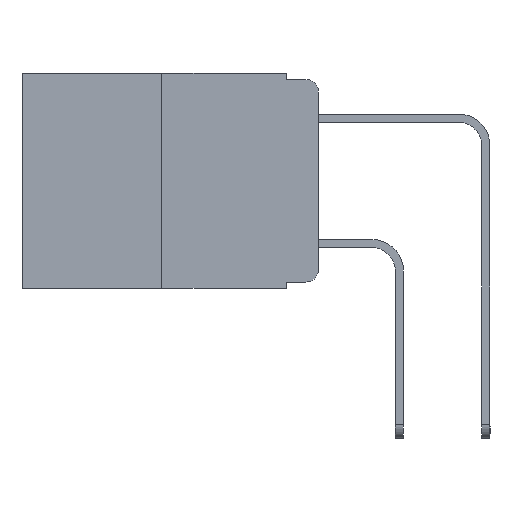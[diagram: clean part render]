
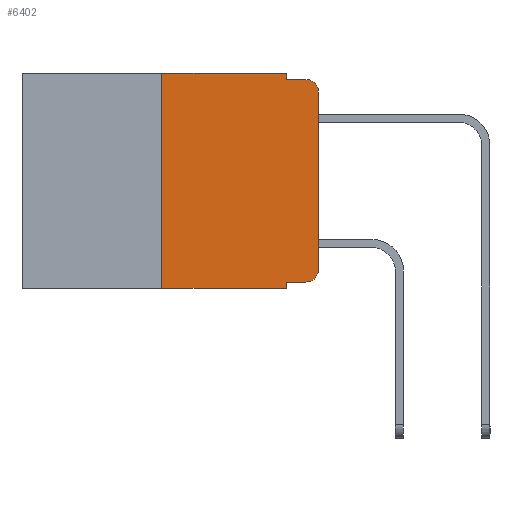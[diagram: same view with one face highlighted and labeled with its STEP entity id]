
A CAD part, left-side view. The second image highlights one B-rep face of the part: STEP entity #6402.
In plain terms, the highlighted planar face has unit normal (-1, 0, 0).
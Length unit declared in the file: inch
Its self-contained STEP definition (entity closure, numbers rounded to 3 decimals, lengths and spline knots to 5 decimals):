
#211 = VERTEX_POINT ( 'NONE', #11814 ) ;
#403 = ORIENTED_EDGE ( 'NONE', *, *, #9901, .F. ) ;
#454 = CARTESIAN_POINT ( 'NONE',  ( 0., 0.051, -0.333 ) ) ;
#734 = DIRECTION ( 'NONE',  ( -1., 0., 0. ) ) ;
#766 = EDGE_CURVE ( 'NONE', #15834, #3114, #13687, .T. ) ;
#1026 = VECTOR ( 'NONE', #3762, 39.37008 ) ;
#1349 = VECTOR ( 'NONE', #5720, 39.37008 ) ;
#1378 = CARTESIAN_POINT ( 'NONE',  ( 0., 0., -0.03 ) ) ;
#1543 = DIRECTION ( 'NONE',  ( -1., 0., 0. ) ) ;
#2592 = VERTEX_POINT ( 'NONE', #6957 ) ;
#2936 = ORIENTED_EDGE ( 'NONE', *, *, #7957, .F. ) ;
#3085 = DIRECTION ( 'NONE',  ( 1., 0., 0. ) ) ;
#3114 = VERTEX_POINT ( 'NONE', #5483 ) ;
#3618 = VERTEX_POINT ( 'NONE', #7188 ) ;
#3762 = DIRECTION ( 'NONE',  ( 0., 0., 1. ) ) ;
#3896 = VECTOR ( 'NONE', #9650, 39.37008 ) ;
#3955 = EDGE_CURVE ( 'NONE', #3114, #6745, #17941, .T. ) ;
#4004 = EDGE_CURVE ( 'NONE', #13956, #15834, #19789, .T. ) ;
#4107 = DIRECTION ( 'NONE',  ( 0., 0., 1. ) ) ;
#4834 = CARTESIAN_POINT ( 'NONE',  ( 0., 0.02, -0.03 ) ) ;
#5006 = VERTEX_POINT ( 'NONE', #10937 ) ;
#5483 = CARTESIAN_POINT ( 'NONE',  ( 0., 0., -0.313 ) ) ;
#5720 = DIRECTION ( 'NONE',  ( 0., -1., 0. ) ) ;
#5876 = ORIENTED_EDGE ( 'NONE', *, *, #15227, .F. ) ;
#6144 = EDGE_CURVE ( 'NONE', #3618, #10780, #10019, .T. ) ;
#6225 = ORIENTED_EDGE ( 'NONE', *, *, #6144, .T. ) ;
#6402 = ADVANCED_FACE ( 'NONE', ( #9275 ), #20260, .F. ) ;
#6668 = AXIS2_PLACEMENT_3D ( 'NONE', #4834, #1543, #14152 ) ;
#6745 = VERTEX_POINT ( 'NONE', #1378 ) ;
#6957 = CARTESIAN_POINT ( 'NONE',  ( 0., 0.25, 0. ) ) ;
#7032 = ORIENTED_EDGE ( 'NONE', *, *, #3955, .T. ) ;
#7151 = CARTESIAN_POINT ( 'NONE',  ( 0., 0.051, -0.343 ) ) ;
#7162 = CARTESIAN_POINT ( 'NONE',  ( 0., 0.051, -0.333 ) ) ;
#7188 = CARTESIAN_POINT ( 'NONE',  ( 0., 0.25, -0.343 ) ) ;
#7580 = CARTESIAN_POINT ( 'NONE',  ( 0., 0.051, 0. ) ) ;
#7642 = CIRCLE ( 'NONE', #6668, 0.02 ) ;
#7763 = ORIENTED_EDGE ( 'NONE', *, *, #17057, .F. ) ;
#7957 = EDGE_CURVE ( 'NONE', #211, #5006, #18241, .T. ) ;
#8257 = VECTOR ( 'NONE', #8454, 39.37008 ) ;
#8454 = DIRECTION ( 'NONE',  ( 0., -1., 0. ) ) ;
#8657 = CARTESIAN_POINT ( 'NONE',  ( 0., 0.473, 0. ) ) ;
#9275 = FACE_OUTER_BOUND ( 'NONE', #9461, .T. ) ;
#9461 = EDGE_LOOP ( 'NONE', ( #7032, #16807, #2936, #19501, #403, #5876, #6225, #7763, #18917, #9912 ) ) ;
#9650 = DIRECTION ( 'NONE',  ( 0., 0., -1. ) ) ;
#9901 = EDGE_CURVE ( 'NONE', #2592, #14738, #19431, .T. ) ;
#9912 = ORIENTED_EDGE ( 'NONE', *, *, #766, .T. ) ;
#10019 = LINE ( 'NONE', #19439, #10185 ) ;
#10185 = VECTOR ( 'NONE', #14489, 39.37008 ) ;
#10679 = CARTESIAN_POINT ( 'NONE',  ( 0., 0.051, -0.01 ) ) ;
#10780 = VERTEX_POINT ( 'NONE', #7151 ) ;
#10937 = CARTESIAN_POINT ( 'NONE',  ( 0., 0.02, -0.01 ) ) ;
#11277 = CARTESIAN_POINT ( 'NONE',  ( 0., 0.02, -0.333 ) ) ;
#11814 = CARTESIAN_POINT ( 'NONE',  ( 0., 0.051, -0.01 ) ) ;
#12281 = CARTESIAN_POINT ( 'NONE',  ( 0., 0.25, 0. ) ) ;
#12687 = AXIS2_PLACEMENT_3D ( 'NONE', #13659, #734, #19656 ) ;
#12873 = EDGE_CURVE ( 'NONE', #6745, #5006, #7642, .T. ) ;
#13001 = VECTOR ( 'NONE', #13585, 39.37008 ) ;
#13506 = DIRECTION ( 'NONE',  ( 0., 0., -1. ) ) ;
#13585 = DIRECTION ( 'NONE',  ( 0., -1., 0. ) ) ;
#13659 = CARTESIAN_POINT ( 'NONE',  ( 0., 0.02, -0.313 ) ) ;
#13687 = CIRCLE ( 'NONE', #12687, 0.02 ) ;
#13956 = VERTEX_POINT ( 'NONE', #454 ) ;
#14152 = DIRECTION ( 'NONE',  ( 0., 0., -1. ) ) ;
#14433 = CARTESIAN_POINT ( 'NONE',  ( 0., 0.051, 0. ) ) ;
#14489 = DIRECTION ( 'NONE',  ( 0., -1., 0. ) ) ;
#14738 = VERTEX_POINT ( 'NONE', #16021 ) ;
#15227 = EDGE_CURVE ( 'NONE', #3618, #2592, #16741, .T. ) ;
#15397 = DIRECTION ( 'NONE',  ( 0., 0., -1. ) ) ;
#15834 = VERTEX_POINT ( 'NONE', #11277 ) ;
#16021 = CARTESIAN_POINT ( 'NONE',  ( 0., 0.051, 0. ) ) ;
#16741 = LINE ( 'NONE', #12281, #18035 ) ;
#16807 = ORIENTED_EDGE ( 'NONE', *, *, #12873, .T. ) ;
#17057 = EDGE_CURVE ( 'NONE', #13956, #10780, #18372, .T. ) ;
#17173 = EDGE_CURVE ( 'NONE', #14738, #211, #18667, .T. ) ;
#17941 = LINE ( 'NONE', #19281, #1026 ) ;
#18035 = VECTOR ( 'NONE', #4107, 39.37008 ) ;
#18241 = LINE ( 'NONE', #10679, #13001 ) ;
#18372 = LINE ( 'NONE', #7580, #19097 ) ;
#18667 = LINE ( 'NONE', #14433, #3896 ) ;
#18917 = ORIENTED_EDGE ( 'NONE', *, *, #4004, .T. ) ;
#19097 = VECTOR ( 'NONE', #13506, 39.37008 ) ;
#19281 = CARTESIAN_POINT ( 'NONE',  ( 0., 0., 0. ) ) ;
#19431 = LINE ( 'NONE', #8657, #8257 ) ;
#19436 = AXIS2_PLACEMENT_3D ( 'NONE', #20047, #3085, #15397 ) ;
#19439 = CARTESIAN_POINT ( 'NONE',  ( 0., 0.473, -0.343 ) ) ;
#19501 = ORIENTED_EDGE ( 'NONE', *, *, #17173, .F. ) ;
#19656 = DIRECTION ( 'NONE',  ( 0., 0., -1. ) ) ;
#19789 = LINE ( 'NONE', #7162, #1349 ) ;
#20047 = CARTESIAN_POINT ( 'NONE',  ( 0., 0.473, 0. ) ) ;
#20260 = PLANE ( 'NONE',  #19436 ) ;
